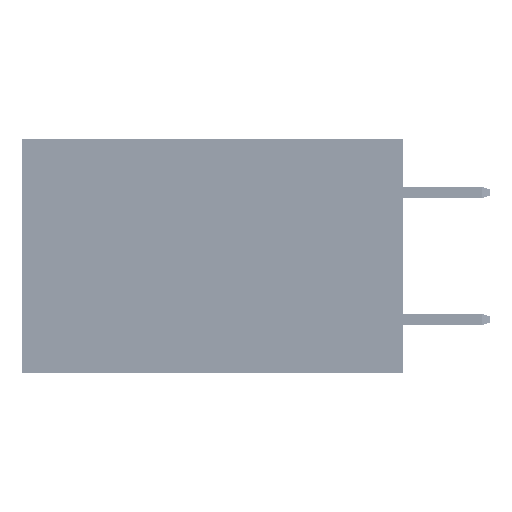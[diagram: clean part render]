
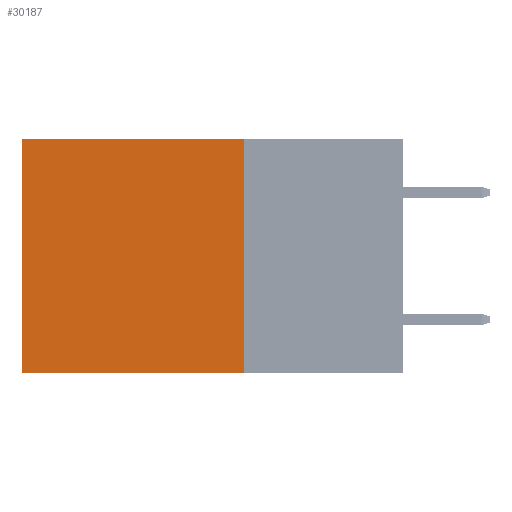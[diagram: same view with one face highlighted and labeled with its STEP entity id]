
A CAD part, left-side view. The second image highlights one B-rep face of the part: STEP entity #30187.
In plain terms, the highlighted planar face has unit normal (-1, 0, 0).
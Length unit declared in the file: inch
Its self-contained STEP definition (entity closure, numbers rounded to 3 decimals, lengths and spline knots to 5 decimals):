
#2480 = AXIS2_PLACEMENT_3D ( 'NONE', #5739, #16032, #46722 ) ;
#5651 = VECTOR ( 'NONE', #39411, 39.37008 ) ;
#5739 = CARTESIAN_POINT ( 'NONE',  ( 0.2875, 0.25, 0. ) ) ;
#9033 = LINE ( 'NONE', #44001, #11524 ) ;
#10447 = LINE ( 'NONE', #20940, #16942 ) ;
#11524 = VECTOR ( 'NONE', #47745, 39.37008 ) ;
#13234 = FACE_OUTER_BOUND ( 'NONE', #38685, .T. ) ;
#15592 = EDGE_CURVE ( 'NONE', #45547, #46119, #21429, .T. ) ;
#15764 = CARTESIAN_POINT ( 'NONE',  ( 0.2875, 0.25, 0. ) ) ;
#16032 = DIRECTION ( 'NONE',  ( 1., 0., 0. ) ) ;
#16096 = VERTEX_POINT ( 'NONE', #29108 ) ;
#16942 = VECTOR ( 'NONE', #40415, 39.37008 ) ;
#19046 = ORIENTED_EDGE ( 'NONE', *, *, #34502, .F. ) ;
#19716 = VECTOR ( 'NONE', #32666, 39.37008 ) ;
#20940 = CARTESIAN_POINT ( 'NONE',  ( 0.2875, 0.6, 0. ) ) ;
#21429 = LINE ( 'NONE', #43928, #19716 ) ;
#27930 = ORIENTED_EDGE ( 'NONE', *, *, #39284, .T. ) ;
#29108 = CARTESIAN_POINT ( 'NONE',  ( 0.2875, 0.6, -0.37 ) ) ;
#30187 = ADVANCED_FACE ( 'NONE', ( #13234 ), #43706, .F. ) ;
#31737 = EDGE_CURVE ( 'NONE', #36157, #16096, #10447, .T. ) ;
#32666 = DIRECTION ( 'NONE',  ( 0., 0., -1. ) ) ;
#34502 = EDGE_CURVE ( 'NONE', #46119, #16096, #9033, .T. ) ;
#36157 = VERTEX_POINT ( 'NONE', #43631 ) ;
#36624 = CARTESIAN_POINT ( 'NONE',  ( 0.2875, 0.25, -0.37 ) ) ;
#38685 = EDGE_LOOP ( 'NONE', ( #43301, #19046, #44460, #27930 ) ) ;
#39284 = EDGE_CURVE ( 'NONE', #45547, #36157, #46674, .T. ) ;
#39411 = DIRECTION ( 'NONE',  ( 0., 1., 0. ) ) ;
#40415 = DIRECTION ( 'NONE',  ( 0., 0., -1. ) ) ;
#43301 = ORIENTED_EDGE ( 'NONE', *, *, #31737, .T. ) ;
#43631 = CARTESIAN_POINT ( 'NONE',  ( 0.2875, 0.6, 0. ) ) ;
#43706 = PLANE ( 'NONE',  #2480 ) ;
#43928 = CARTESIAN_POINT ( 'NONE',  ( 0.2875, 0.25, 0. ) ) ;
#44001 = CARTESIAN_POINT ( 'NONE',  ( 0.2875, 0.25, -0.37 ) ) ;
#44460 = ORIENTED_EDGE ( 'NONE', *, *, #15592, .F. ) ;
#45547 = VERTEX_POINT ( 'NONE', #15764 ) ;
#46119 = VERTEX_POINT ( 'NONE', #36624 ) ;
#46674 = LINE ( 'NONE', #47646, #5651 ) ;
#46722 = DIRECTION ( 'NONE',  ( 0., 0., -1. ) ) ;
#47646 = CARTESIAN_POINT ( 'NONE',  ( 0.2875, 0.25, 0. ) ) ;
#47745 = DIRECTION ( 'NONE',  ( 0., 1., 0. ) ) ;
